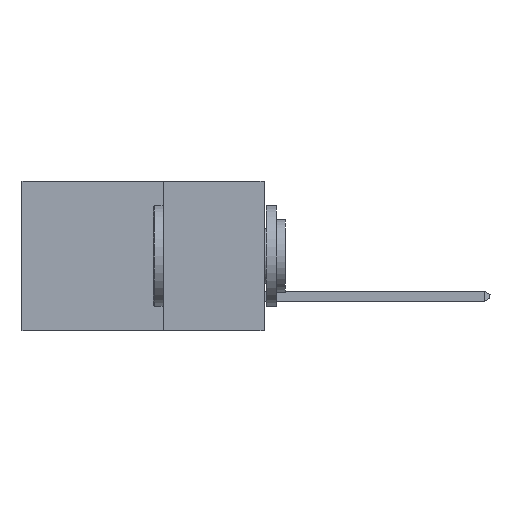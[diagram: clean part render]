
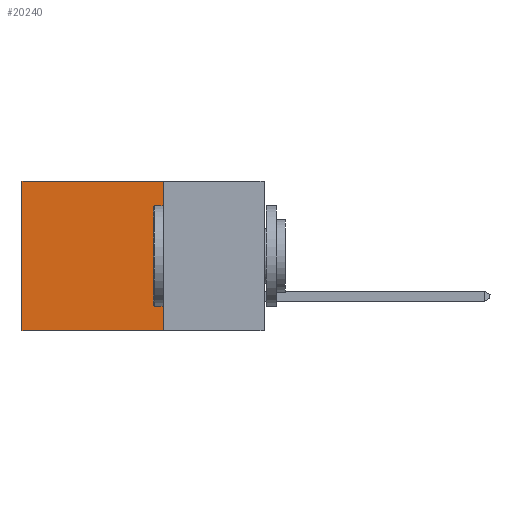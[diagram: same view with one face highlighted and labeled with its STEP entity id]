
A CAD part, left-side view. The second image highlights one B-rep face of the part: STEP entity #20240.
In plain terms, the highlighted planar face has unit normal (-1, 0, 0).
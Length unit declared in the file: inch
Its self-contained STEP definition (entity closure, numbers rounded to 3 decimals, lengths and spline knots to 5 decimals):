
#46 = ORIENTED_EDGE ( 'NONE', *, *, #2456, .F. ) ;
#403 = DIRECTION ( 'NONE',  ( 0., 0., -1. ) ) ;
#1636 = CARTESIAN_POINT ( 'NONE',  ( 0.2615, 0.25, -0.37 ) ) ;
#2456 = EDGE_CURVE ( 'NONE', #5115, #15133, #9171, .T. ) ;
#2698 = DIRECTION ( 'NONE',  ( 0., 1., 0. ) ) ;
#4126 = ORIENTED_EDGE ( 'NONE', *, *, #13024, .T. ) ;
#4465 = VERTEX_POINT ( 'NONE', #16385 ) ;
#4596 = PLANE ( 'NONE',  #17526 ) ;
#5067 = ORIENTED_EDGE ( 'NONE', *, *, #14522, .F. ) ;
#5115 = VERTEX_POINT ( 'NONE', #7168 ) ;
#6084 = LINE ( 'NONE', #17302, #15232 ) ;
#6283 = DIRECTION ( 'NONE',  ( 0., 0., -1. ) ) ;
#7168 = CARTESIAN_POINT ( 'NONE',  ( 0.2615, 0.25, -0.37 ) ) ;
#7991 = EDGE_CURVE ( 'NONE', #4465, #13925, #6084, .T. ) ;
#8000 = DIRECTION ( 'NONE',  ( 1., 0., 0. ) ) ;
#9171 = LINE ( 'NONE', #15685, #14676 ) ;
#9447 = DIRECTION ( 'NONE',  ( 0., 0., -1. ) ) ;
#11524 = FACE_OUTER_BOUND ( 'NONE', #18216, .T. ) ;
#11544 = CARTESIAN_POINT ( 'NONE',  ( 0.2615, 0.6, -0.37 ) ) ;
#12653 = LINE ( 'NONE', #1636, #18778 ) ;
#13024 = EDGE_CURVE ( 'NONE', #13925, #15133, #16719, .T. ) ;
#13637 = VECTOR ( 'NONE', #403, 39.37008 ) ;
#13670 = DIRECTION ( 'NONE',  ( 0., 1., 0. ) ) ;
#13925 = VERTEX_POINT ( 'NONE', #14965 ) ;
#14522 = EDGE_CURVE ( 'NONE', #4465, #5115, #12653, .T. ) ;
#14676 = VECTOR ( 'NONE', #13670, 39.37008 ) ;
#14819 = ORIENTED_EDGE ( 'NONE', *, *, #7991, .T. ) ;
#14965 = CARTESIAN_POINT ( 'NONE',  ( 0.2615, 0.6, 0. ) ) ;
#15133 = VERTEX_POINT ( 'NONE', #11544 ) ;
#15232 = VECTOR ( 'NONE', #2698, 39.37008 ) ;
#15685 = CARTESIAN_POINT ( 'NONE',  ( 0.2615, 0.25, -0.37 ) ) ;
#16322 = CARTESIAN_POINT ( 'NONE',  ( 0.2615, 0.25, -0.37 ) ) ;
#16385 = CARTESIAN_POINT ( 'NONE',  ( 0.2615, 0.25, 0. ) ) ;
#16719 = LINE ( 'NONE', #19598, #13637 ) ;
#17302 = CARTESIAN_POINT ( 'NONE',  ( 0.2615, 0.25, 0. ) ) ;
#17526 = AXIS2_PLACEMENT_3D ( 'NONE', #16322, #8000, #6283 ) ;
#18216 = EDGE_LOOP ( 'NONE', ( #4126, #46, #5067, #14819 ) ) ;
#18778 = VECTOR ( 'NONE', #9447, 39.37008 ) ;
#19598 = CARTESIAN_POINT ( 'NONE',  ( 0.2615, 0.6, -0.37 ) ) ;
#20240 = ADVANCED_FACE ( 'NONE', ( #11524 ), #4596, .F. ) ;
